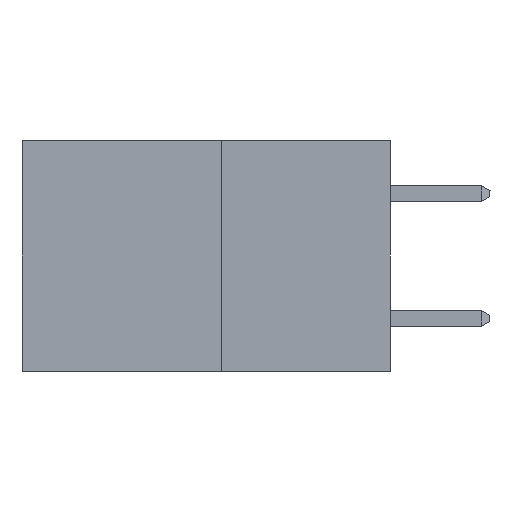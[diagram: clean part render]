
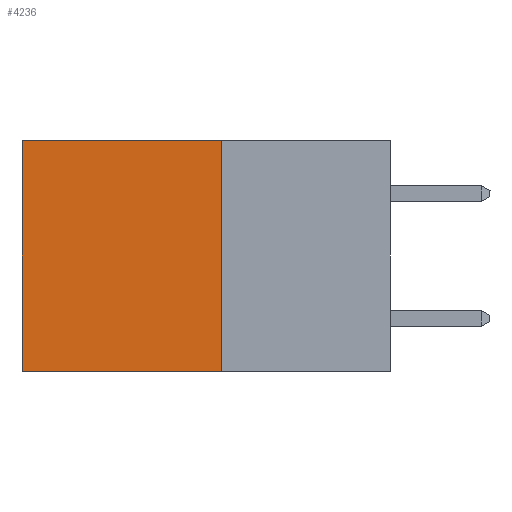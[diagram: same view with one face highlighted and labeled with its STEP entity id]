
A CAD part, left-side view. The second image highlights one B-rep face of the part: STEP entity #4236.
In plain terms, the highlighted planar face has unit normal (-1, 0, 0).
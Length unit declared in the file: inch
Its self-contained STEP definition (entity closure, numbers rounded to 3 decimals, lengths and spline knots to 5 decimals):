
#384 = EDGE_CURVE ( 'NONE', #12952, #10868, #7654, .T. ) ;
#724 = EDGE_CURVE ( 'NONE', #10868, #9461, #14950, .T. ) ;
#2410 = CARTESIAN_POINT ( 'NONE',  ( 0.277, 0.27, -0.37 ) ) ;
#2614 = PLANE ( 'NONE',  #9305 ) ;
#3645 = EDGE_LOOP ( 'NONE', ( #17472, #13988, #16477, #15027 ) ) ;
#4236 = ADVANCED_FACE ( 'NONE', ( #18627 ), #2614, .F. ) ;
#5917 = LINE ( 'NONE', #5926, #14509 ) ;
#5926 = CARTESIAN_POINT ( 'NONE',  ( 0.277, 0.27, -0.37 ) ) ;
#6142 = EDGE_CURVE ( 'NONE', #10641, #9461, #7716, .T. ) ;
#7503 = DIRECTION ( 'NONE',  ( 0., 0., -1. ) ) ;
#7654 = LINE ( 'NONE', #9217, #16246 ) ;
#7716 = LINE ( 'NONE', #2410, #11502 ) ;
#9046 = CARTESIAN_POINT ( 'NONE',  ( 0.277, 0.27, -0.37 ) ) ;
#9217 = CARTESIAN_POINT ( 'NONE',  ( 0.277, 0.27, 0. ) ) ;
#9305 = AXIS2_PLACEMENT_3D ( 'NONE', #9046, #17175, #7503 ) ;
#9461 = VERTEX_POINT ( 'NONE', #18186 ) ;
#10641 = VERTEX_POINT ( 'NONE', #19349 ) ;
#10868 = VERTEX_POINT ( 'NONE', #15013 ) ;
#11502 = VECTOR ( 'NONE', #15338, 39.37008 ) ;
#12952 = VERTEX_POINT ( 'NONE', #15304 ) ;
#13988 = ORIENTED_EDGE ( 'NONE', *, *, #6142, .F. ) ;
#14509 = VECTOR ( 'NONE', #17240, 39.37008 ) ;
#14950 = LINE ( 'NONE', #15134, #18759 ) ;
#15013 = CARTESIAN_POINT ( 'NONE',  ( 0.277, 0.59, 0. ) ) ;
#15027 = ORIENTED_EDGE ( 'NONE', *, *, #384, .T. ) ;
#15134 = CARTESIAN_POINT ( 'NONE',  ( 0.277, 0.59, -0.37 ) ) ;
#15304 = CARTESIAN_POINT ( 'NONE',  ( 0.277, 0.27, 0. ) ) ;
#15338 = DIRECTION ( 'NONE',  ( 0., 1., 0. ) ) ;
#16246 = VECTOR ( 'NONE', #20521, 39.37008 ) ;
#16477 = ORIENTED_EDGE ( 'NONE', *, *, #18493, .F. ) ;
#16781 = DIRECTION ( 'NONE',  ( 0., 0., -1. ) ) ;
#17175 = DIRECTION ( 'NONE',  ( 1., 0., 0. ) ) ;
#17240 = DIRECTION ( 'NONE',  ( 0., 0., -1. ) ) ;
#17472 = ORIENTED_EDGE ( 'NONE', *, *, #724, .T. ) ;
#18186 = CARTESIAN_POINT ( 'NONE',  ( 0.277, 0.59, -0.37 ) ) ;
#18493 = EDGE_CURVE ( 'NONE', #12952, #10641, #5917, .T. ) ;
#18627 = FACE_OUTER_BOUND ( 'NONE', #3645, .T. ) ;
#18759 = VECTOR ( 'NONE', #16781, 39.37008 ) ;
#19349 = CARTESIAN_POINT ( 'NONE',  ( 0.277, 0.27, -0.37 ) ) ;
#20521 = DIRECTION ( 'NONE',  ( 0., 1., 0. ) ) ;
